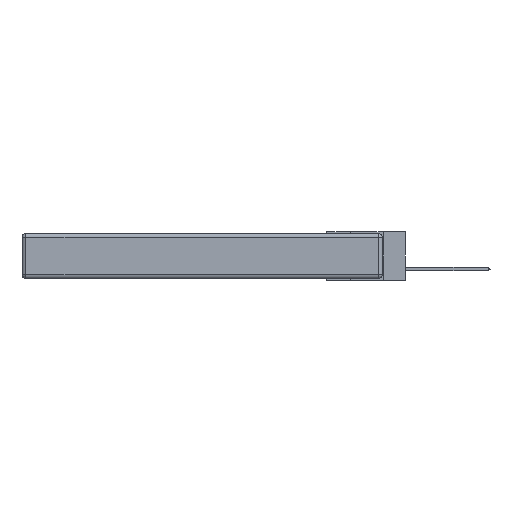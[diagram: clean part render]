
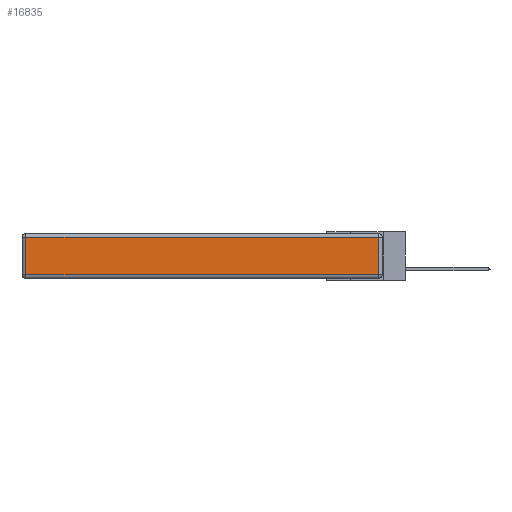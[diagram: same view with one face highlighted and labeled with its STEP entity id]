
A CAD part, left-side view. The second image highlights one B-rep face of the part: STEP entity #16835.
In plain terms, the highlighted planar face has unit normal (-1, 0, 0).
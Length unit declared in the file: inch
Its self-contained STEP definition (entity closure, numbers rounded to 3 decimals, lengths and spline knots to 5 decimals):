
#416 = EDGE_CURVE ( 'NONE', #716, #25412, #7812, .T. ) ;
#716 = VERTEX_POINT ( 'NONE', #1955 ) ;
#1955 = CARTESIAN_POINT ( 'NONE',  ( 0., 0.03, -0.03 ) ) ;
#2475 = VERTEX_POINT ( 'NONE', #25616 ) ;
#3736 = CARTESIAN_POINT ( 'NONE',  ( 0., 0.03, -0.343 ) ) ;
#5803 = VECTOR ( 'NONE', #26518, 39.37008 ) ;
#6450 = PLANE ( 'NONE',  #20036 ) ;
#6617 = DIRECTION ( 'NONE',  ( 0., 0., 1. ) ) ;
#7380 = VECTOR ( 'NONE', #19116, 39.37008 ) ;
#7756 = EDGE_CURVE ( 'NONE', #25412, #19242, #14126, .T. ) ;
#7812 = LINE ( 'NONE', #13405, #11690 ) ;
#7932 = ORIENTED_EDGE ( 'NONE', *, *, #416, .T. ) ;
#9618 = LINE ( 'NONE', #17047, #7380 ) ;
#10081 = CARTESIAN_POINT ( 'NONE',  ( 0., 2.72, -0.03 ) ) ;
#11690 = VECTOR ( 'NONE', #17680, 39.37008 ) ;
#12785 = VECTOR ( 'NONE', #20322, 39.37008 ) ;
#13255 = EDGE_CURVE ( 'NONE', #2475, #716, #22778, .T. ) ;
#13405 = CARTESIAN_POINT ( 'NONE',  ( 0., 2.75, -0.03 ) ) ;
#14126 = LINE ( 'NONE', #24275, #5803 ) ;
#14599 = CARTESIAN_POINT ( 'NONE',  ( 0., 2.72, -0.313 ) ) ;
#14689 = DIRECTION ( 'NONE',  ( -1., 0., 0. ) ) ;
#16783 = CARTESIAN_POINT ( 'NONE',  ( 0., 0., -0.343 ) ) ;
#16835 = ADVANCED_FACE ( 'NONE', ( #22301 ), #6450, .T. ) ;
#17047 = CARTESIAN_POINT ( 'NONE',  ( 0., 0., -0.313 ) ) ;
#17680 = DIRECTION ( 'NONE',  ( 0., 1., 0. ) ) ;
#18776 = ORIENTED_EDGE ( 'NONE', *, *, #19364, .T. ) ;
#19116 = DIRECTION ( 'NONE',  ( 0., -1., 0. ) ) ;
#19242 = VERTEX_POINT ( 'NONE', #14599 ) ;
#19364 = EDGE_CURVE ( 'NONE', #19242, #2475, #9618, .T. ) ;
#20036 = AXIS2_PLACEMENT_3D ( 'NONE', #16783, #14689, #6617 ) ;
#20322 = DIRECTION ( 'NONE',  ( 0., 0., 1. ) ) ;
#21978 = ORIENTED_EDGE ( 'NONE', *, *, #7756, .T. ) ;
#22301 = FACE_OUTER_BOUND ( 'NONE', #25764, .T. ) ;
#22778 = LINE ( 'NONE', #3736, #12785 ) ;
#24275 = CARTESIAN_POINT ( 'NONE',  ( 0., 2.72, -0.343 ) ) ;
#24898 = ORIENTED_EDGE ( 'NONE', *, *, #13255, .T. ) ;
#25412 = VERTEX_POINT ( 'NONE', #10081 ) ;
#25616 = CARTESIAN_POINT ( 'NONE',  ( 0., 0.03, -0.313 ) ) ;
#25764 = EDGE_LOOP ( 'NONE', ( #18776, #24898, #7932, #21978 ) ) ;
#26518 = DIRECTION ( 'NONE',  ( 0., 0., -1. ) ) ;
